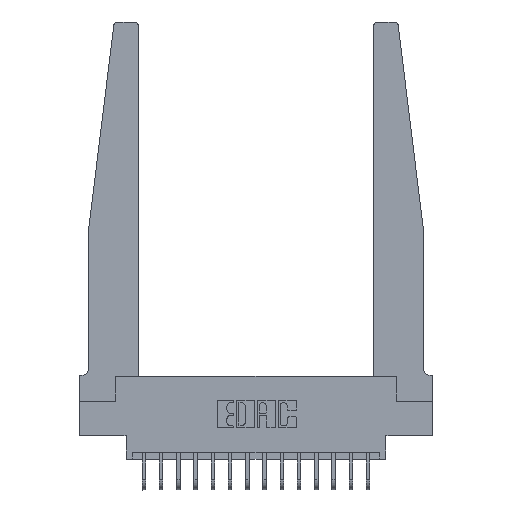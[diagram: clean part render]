
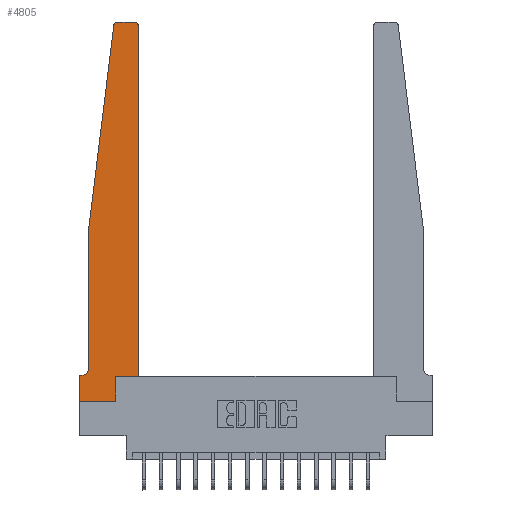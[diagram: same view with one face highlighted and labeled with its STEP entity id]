
A CAD part, top view. The second image highlights one B-rep face of the part: STEP entity #4805.
In plain terms, the highlighted planar face has unit normal (0, 0, 1).
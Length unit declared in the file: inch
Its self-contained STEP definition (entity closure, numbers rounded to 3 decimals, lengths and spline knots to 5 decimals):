
#83 = VERTEX_POINT ( 'NONE', #9359 ) ;
#321 = ORIENTED_EDGE ( 'NONE', *, *, #956, .T. ) ;
#401 = LINE ( 'NONE', #11369, #6956 ) ;
#453 = VERTEX_POINT ( 'NONE', #4848 ) ;
#565 = VERTEX_POINT ( 'NONE', #11148 ) ;
#733 = EDGE_CURVE ( 'NONE', #10949, #7143, #11551, .T. ) ;
#739 = VERTEX_POINT ( 'NONE', #8884 ) ;
#956 = EDGE_CURVE ( 'NONE', #739, #17504, #10166, .T. ) ;
#1168 = CARTESIAN_POINT ( 'NONE',  ( 0.065, 1.25, 0.37 ) ) ;
#1753 = ORIENTED_EDGE ( 'NONE', *, *, #11420, .T. ) ;
#1980 = ORIENTED_EDGE ( 'NONE', *, *, #8211, .T. ) ;
#2377 = PLANE ( 'NONE',  #9196 ) ;
#2413 = VECTOR ( 'NONE', #16785, 39.37008 ) ;
#2644 = DIRECTION ( 'NONE',  ( 1., 0., 0. ) ) ;
#3181 = VERTEX_POINT ( 'NONE', #9733 ) ;
#3488 = DIRECTION ( 'NONE',  ( 1., 0., 0. ) ) ;
#3492 = AXIS2_PLACEMENT_3D ( 'NONE', #17385, #12830, #3488 ) ;
#3827 = CARTESIAN_POINT ( 'NONE',  ( 0.25, 2.75, 0.37 ) ) ;
#4188 = EDGE_CURVE ( 'NONE', #83, #10851, #4283, .T. ) ;
#4283 = LINE ( 'NONE', #9257, #13402 ) ;
#4805 = ADVANCED_FACE ( 'NONE', ( #10201 ), #2377, .T. ) ;
#4848 = CARTESIAN_POINT ( 'NONE',  ( 0.24675, 2.72367, 0.37 ) ) ;
#5006 = VECTOR ( 'NONE', #15165, 39.37008 ) ;
#5701 = VECTOR ( 'NONE', #19591, 39.37008 ) ;
#5814 = DIRECTION ( 'NONE',  ( 0., 0., -1. ) ) ;
#6008 = CARTESIAN_POINT ( 'NONE',  ( 0.065, 0.2375, 0.37 ) ) ;
#6117 = VECTOR ( 'NONE', #11707, 39.37008 ) ;
#6129 = LINE ( 'NONE', #6221, #14069 ) ;
#6169 = EDGE_CURVE ( 'NONE', #17504, #7450, #18394, .T. ) ;
#6221 = CARTESIAN_POINT ( 'NONE',  ( 0.2605, 0.18, 0.37 ) ) ;
#6448 = CARTESIAN_POINT ( 'NONE',  ( 0.27653, 2.72, 0.37 ) ) ;
#6851 = DIRECTION ( 'NONE',  ( 1., 0., 0. ) ) ;
#6956 = VECTOR ( 'NONE', #18942, 39.37008 ) ;
#7143 = VERTEX_POINT ( 'NONE', #17731 ) ;
#7450 = VERTEX_POINT ( 'NONE', #8068 ) ;
#7652 = ORIENTED_EDGE ( 'NONE', *, *, #14043, .T. ) ;
#7763 = CARTESIAN_POINT ( 'NONE',  ( 0.425, 0.18, 0.37 ) ) ;
#7833 = ORIENTED_EDGE ( 'NONE', *, *, #9814, .T. ) ;
#8068 = CARTESIAN_POINT ( 'NONE',  ( 0.425, 2.72, 0.37 ) ) ;
#8211 = EDGE_CURVE ( 'NONE', #16547, #83, #16389, .T. ) ;
#8470 = DIRECTION ( 'NONE',  ( 0., 0., 1. ) ) ;
#8884 = CARTESIAN_POINT ( 'NONE',  ( 0.2605, 0.18, 0.37 ) ) ;
#9196 = AXIS2_PLACEMENT_3D ( 'NONE', #11737, #8470, #6851 ) ;
#9257 = CARTESIAN_POINT ( 'NONE',  ( 0.065, 0.1875, 0.37 ) ) ;
#9359 = CARTESIAN_POINT ( 'NONE',  ( 0.015, 0.1875, 0.37 ) ) ;
#9488 = ORIENTED_EDGE ( 'NONE', *, *, #4188, .T. ) ;
#9613 = EDGE_CURVE ( 'NONE', #7450, #10949, #19675, .T. ) ;
#9684 = CARTESIAN_POINT ( 'NONE',  ( 0.395, 2.75, 0.37 ) ) ;
#9733 = CARTESIAN_POINT ( 'NONE',  ( 0., 0., 0.37 ) ) ;
#9814 = EDGE_CURVE ( 'NONE', #565, #16547, #19291, .T. ) ;
#10116 = DIRECTION ( 'NONE',  ( -1., 0., 0. ) ) ;
#10122 = ORIENTED_EDGE ( 'NONE', *, *, #733, .T. ) ;
#10166 = LINE ( 'NONE', #16336, #6117 ) ;
#10201 = FACE_OUTER_BOUND ( 'NONE', #10804, .T. ) ;
#10361 = CARTESIAN_POINT ( 'NONE',  ( 0., 0., 0.37 ) ) ;
#10397 = DIRECTION ( 'NONE',  ( -1., 0., 0. ) ) ;
#10804 = EDGE_LOOP ( 'NONE', ( #10122, #16461, #7652, #7833, #1980, #9488, #13088, #1753, #13878, #321, #16590, #11629 ) ) ;
#10828 = EDGE_CURVE ( 'NONE', #18809, #739, #6129, .T. ) ;
#10851 = VERTEX_POINT ( 'NONE', #11218 ) ;
#10949 = VERTEX_POINT ( 'NONE', #9684 ) ;
#11119 = DIRECTION ( 'NONE',  ( 0., 0., 1. ) ) ;
#11148 = CARTESIAN_POINT ( 'NONE',  ( 0.065, 1.25, 0.37 ) ) ;
#11218 = CARTESIAN_POINT ( 'NONE',  ( 0., 0.1875, 0.37 ) ) ;
#11261 = CARTESIAN_POINT ( 'NONE',  ( 0.2605, 0., 0.37 ) ) ;
#11369 = CARTESIAN_POINT ( 'NONE',  ( 0., 0., 0.37 ) ) ;
#11420 = EDGE_CURVE ( 'NONE', #3181, #18809, #19478, .T. ) ;
#11551 = LINE ( 'NONE', #3827, #16795 ) ;
#11629 = ORIENTED_EDGE ( 'NONE', *, *, #9613, .T. ) ;
#11707 = DIRECTION ( 'NONE',  ( 1., 0., 0. ) ) ;
#11737 = CARTESIAN_POINT ( 'NONE',  ( 0., 0.1875, 0.37 ) ) ;
#12120 = DIRECTION ( 'NONE',  ( -1., 0., 0. ) ) ;
#12353 = DIRECTION ( 'NONE',  ( 0., 1., 0. ) ) ;
#12608 = AXIS2_PLACEMENT_3D ( 'NONE', #6448, #11119, #17295 ) ;
#12830 = DIRECTION ( 'NONE',  ( 0., 0., 1. ) ) ;
#13088 = ORIENTED_EDGE ( 'NONE', *, *, #13313, .T. ) ;
#13313 = EDGE_CURVE ( 'NONE', #10851, #3181, #401, .T. ) ;
#13347 = CARTESIAN_POINT ( 'NONE',  ( 0.015, 0.2375, 0.37 ) ) ;
#13402 = VECTOR ( 'NONE', #12120, 39.37008 ) ;
#13878 = ORIENTED_EDGE ( 'NONE', *, *, #10828, .T. ) ;
#14043 = EDGE_CURVE ( 'NONE', #453, #565, #15060, .T. ) ;
#14069 = VECTOR ( 'NONE', #12353, 39.37008 ) ;
#15060 = LINE ( 'NONE', #1168, #5006 ) ;
#15165 = DIRECTION ( 'NONE',  ( -0.122, -0.992, 0. ) ) ;
#16336 = CARTESIAN_POINT ( 'NONE',  ( 0.425, 0.18, 0.37 ) ) ;
#16389 = CIRCLE ( 'NONE', #19303, 0.05 ) ;
#16461 = ORIENTED_EDGE ( 'NONE', *, *, #18082, .T. ) ;
#16547 = VERTEX_POINT ( 'NONE', #6008 ) ;
#16590 = ORIENTED_EDGE ( 'NONE', *, *, #6169, .T. ) ;
#16626 = VECTOR ( 'NONE', #2644, 39.37008 ) ;
#16785 = DIRECTION ( 'NONE',  ( 0., 1., 0. ) ) ;
#16795 = VECTOR ( 'NONE', #10116, 39.37008 ) ;
#17295 = DIRECTION ( 'NONE',  ( 1., 0., 0. ) ) ;
#17385 = CARTESIAN_POINT ( 'NONE',  ( 0.395, 2.72, 0.37 ) ) ;
#17461 = CIRCLE ( 'NONE', #12608, 0.03 ) ;
#17504 = VERTEX_POINT ( 'NONE', #18927 ) ;
#17731 = CARTESIAN_POINT ( 'NONE',  ( 0.27653, 2.75, 0.37 ) ) ;
#18082 = EDGE_CURVE ( 'NONE', #7143, #453, #17461, .T. ) ;
#18394 = LINE ( 'NONE', #7763, #2413 ) ;
#18809 = VERTEX_POINT ( 'NONE', #11261 ) ;
#18927 = CARTESIAN_POINT ( 'NONE',  ( 0.425, 0.18, 0.37 ) ) ;
#18942 = DIRECTION ( 'NONE',  ( 0., -1., 0. ) ) ;
#19291 = LINE ( 'NONE', #19495, #5701 ) ;
#19303 = AXIS2_PLACEMENT_3D ( 'NONE', #13347, #5814, #10397 ) ;
#19478 = LINE ( 'NONE', #10361, #16626 ) ;
#19495 = CARTESIAN_POINT ( 'NONE',  ( 0.065, 1.25, 0.37 ) ) ;
#19591 = DIRECTION ( 'NONE',  ( 0., -1., 0. ) ) ;
#19675 = CIRCLE ( 'NONE', #3492, 0.03 ) ;
